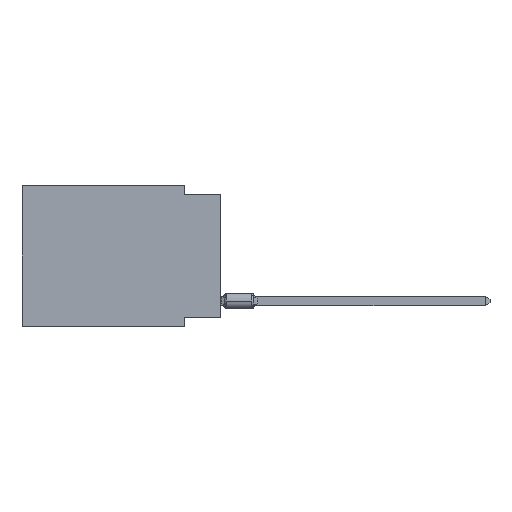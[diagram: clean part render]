
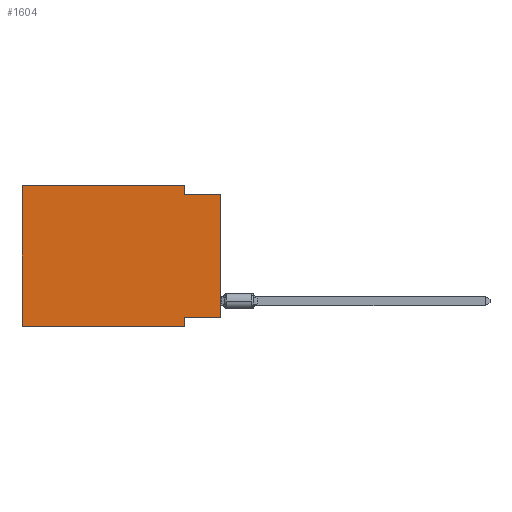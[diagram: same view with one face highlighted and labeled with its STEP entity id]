
A CAD part, left-side view. The second image highlights one B-rep face of the part: STEP entity #1604.
In plain terms, the highlighted planar face has unit normal (-1, 0, 0).
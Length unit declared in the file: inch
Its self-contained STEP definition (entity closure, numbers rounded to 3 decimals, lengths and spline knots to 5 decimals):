
#218 = DIRECTION ( 'NONE',  ( 0., 0., 1. ) ) ;
#1023 = VERTEX_POINT ( 'NONE', #14429 ) ;
#1154 = CARTESIAN_POINT ( 'NONE',  ( 0., 0.55, -0.39 ) ) ;
#1531 = DIRECTION ( 'NONE',  ( 1., 0., 0. ) ) ;
#1604 = ADVANCED_FACE ( 'NONE', ( #3241 ), #7869, .F. ) ;
#1663 = VECTOR ( 'NONE', #6203, 39.37008 ) ;
#2767 = VECTOR ( 'NONE', #3156, 39.37008 ) ;
#3156 = DIRECTION ( 'NONE',  ( 0., -1., 0. ) ) ;
#3241 = FACE_OUTER_BOUND ( 'NONE', #17789, .T. ) ;
#3910 = AXIS2_PLACEMENT_3D ( 'NONE', #22944, #1531, #20830 ) ;
#4458 = CARTESIAN_POINT ( 'NONE',  ( 0., 0.55, 0. ) ) ;
#4511 = ORIENTED_EDGE ( 'NONE', *, *, #25489, .F. ) ;
#4619 = CARTESIAN_POINT ( 'NONE',  ( 0., 0., -0.365 ) ) ;
#5052 = VERTEX_POINT ( 'NONE', #25473 ) ;
#6203 = DIRECTION ( 'NONE',  ( 0., -1., 0. ) ) ;
#6490 = VERTEX_POINT ( 'NONE', #23040 ) ;
#6828 = EDGE_CURVE ( 'NONE', #13444, #7579, #15961, .T. ) ;
#7198 = CARTESIAN_POINT ( 'NONE',  ( 0., 0.1, -0.39 ) ) ;
#7367 = VERTEX_POINT ( 'NONE', #4619 ) ;
#7579 = VERTEX_POINT ( 'NONE', #11211 ) ;
#7869 = PLANE ( 'NONE',  #3910 ) ;
#8379 = LINE ( 'NONE', #4458, #21075 ) ;
#8852 = VECTOR ( 'NONE', #23786, 39.37008 ) ;
#8917 = EDGE_CURVE ( 'NONE', #18793, #1023, #8379, .T. ) ;
#9228 = ORIENTED_EDGE ( 'NONE', *, *, #23543, .T. ) ;
#10165 = VECTOR ( 'NONE', #11408, 39.37008 ) ;
#10488 = ORIENTED_EDGE ( 'NONE', *, *, #6828, .F. ) ;
#10906 = ORIENTED_EDGE ( 'NONE', *, *, #25773, .F. ) ;
#10909 = VECTOR ( 'NONE', #22335, 39.37008 ) ;
#11018 = LINE ( 'NONE', #24685, #16713 ) ;
#11211 = CARTESIAN_POINT ( 'NONE',  ( 0., 0., -0.025 ) ) ;
#11408 = DIRECTION ( 'NONE',  ( 0., 0., -1. ) ) ;
#11750 = DIRECTION ( 'NONE',  ( 0., 1., 0. ) ) ;
#11858 = CARTESIAN_POINT ( 'NONE',  ( 0., 0., -0.025 ) ) ;
#11971 = VECTOR ( 'NONE', #11750, 39.37008 ) ;
#12391 = ORIENTED_EDGE ( 'NONE', *, *, #27431, .T. ) ;
#13444 = VERTEX_POINT ( 'NONE', #18064 ) ;
#13745 = CARTESIAN_POINT ( 'NONE',  ( 0., 0., 0. ) ) ;
#14429 = CARTESIAN_POINT ( 'NONE',  ( 0., 0.55, 0. ) ) ;
#15961 = LINE ( 'NONE', #11858, #2767 ) ;
#16129 = CARTESIAN_POINT ( 'NONE',  ( 0., 0., -0.365 ) ) ;
#16400 = LINE ( 'NONE', #16129, #11971 ) ;
#16713 = VECTOR ( 'NONE', #27079, 39.37008 ) ;
#16940 = EDGE_CURVE ( 'NONE', #7367, #6490, #16400, .T. ) ;
#17181 = LINE ( 'NONE', #21256, #1663 ) ;
#17789 = EDGE_LOOP ( 'NONE', ( #9228, #10488, #26288, #10906, #24618, #12391, #4511, #24490 ) ) ;
#18064 = CARTESIAN_POINT ( 'NONE',  ( 0., 0.1, -0.025 ) ) ;
#18793 = VERTEX_POINT ( 'NONE', #1154 ) ;
#20017 = LINE ( 'NONE', #7198, #10165 ) ;
#20344 = LINE ( 'NONE', #13745, #10909 ) ;
#20830 = DIRECTION ( 'NONE',  ( 0., 0., -1. ) ) ;
#21075 = VECTOR ( 'NONE', #218, 39.37008 ) ;
#21256 = CARTESIAN_POINT ( 'NONE',  ( 0., 0.55, 0. ) ) ;
#21545 = CARTESIAN_POINT ( 'NONE',  ( 0., 0.1, -0.39 ) ) ;
#22276 = EDGE_CURVE ( 'NONE', #5052, #13444, #11018, .T. ) ;
#22335 = DIRECTION ( 'NONE',  ( 0., 0., 1. ) ) ;
#22944 = CARTESIAN_POINT ( 'NONE',  ( 0., 0.55, 0. ) ) ;
#23040 = CARTESIAN_POINT ( 'NONE',  ( 0., 0.1, -0.365 ) ) ;
#23357 = CARTESIAN_POINT ( 'NONE',  ( 0., 0.55, -0.39 ) ) ;
#23543 = EDGE_CURVE ( 'NONE', #7367, #7579, #20344, .T. ) ;
#23786 = DIRECTION ( 'NONE',  ( 0., -1., 0. ) ) ;
#24490 = ORIENTED_EDGE ( 'NONE', *, *, #16940, .F. ) ;
#24618 = ORIENTED_EDGE ( 'NONE', *, *, #8917, .F. ) ;
#24685 = CARTESIAN_POINT ( 'NONE',  ( 0., 0.1, 0. ) ) ;
#25473 = CARTESIAN_POINT ( 'NONE',  ( 0., 0.1, 0. ) ) ;
#25489 = EDGE_CURVE ( 'NONE', #6490, #25883, #20017, .T. ) ;
#25773 = EDGE_CURVE ( 'NONE', #1023, #5052, #17181, .T. ) ;
#25883 = VERTEX_POINT ( 'NONE', #21545 ) ;
#26050 = LINE ( 'NONE', #23357, #8852 ) ;
#26288 = ORIENTED_EDGE ( 'NONE', *, *, #22276, .F. ) ;
#27079 = DIRECTION ( 'NONE',  ( 0., 0., -1. ) ) ;
#27431 = EDGE_CURVE ( 'NONE', #18793, #25883, #26050, .T. ) ;
